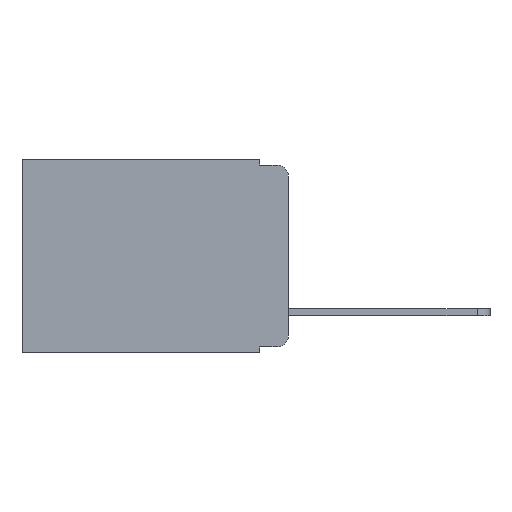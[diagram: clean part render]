
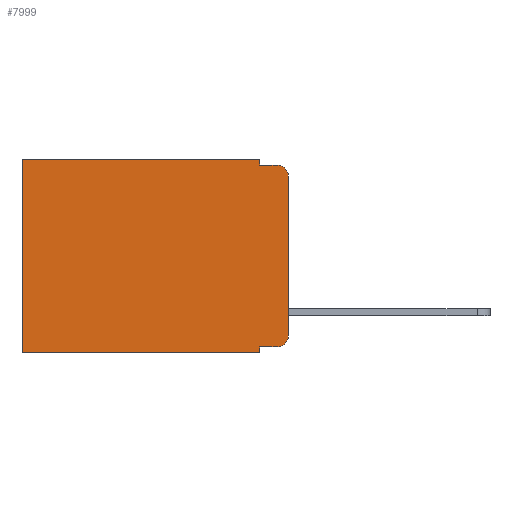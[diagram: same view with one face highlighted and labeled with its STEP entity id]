
A CAD part, left-side view. The second image highlights one B-rep face of the part: STEP entity #7999.
In plain terms, the highlighted planar face has unit normal (-1, 0, 0).
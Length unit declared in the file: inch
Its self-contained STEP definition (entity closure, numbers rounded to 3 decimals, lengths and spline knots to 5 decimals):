
#23 = CARTESIAN_POINT ( 'NONE',  ( 0.298, 0.051, 0. ) ) ;
#104 = EDGE_CURVE ( 'NONE', #6155, #2295, #5084, .T. ) ;
#171 = LINE ( 'NONE', #7430, #8221 ) ;
#211 = EDGE_CURVE ( 'NONE', #7079, #8938, #4301, .T. ) ;
#266 = DIRECTION ( 'NONE',  ( 0., 0., -1. ) ) ;
#279 = EDGE_CURVE ( 'NONE', #7079, #2295, #1635, .T. ) ;
#537 = AXIS2_PLACEMENT_3D ( 'NONE', #9211, #1673, #1945 ) ;
#915 = CARTESIAN_POINT ( 'NONE',  ( 0.298, 0.473, 0. ) ) ;
#1089 = AXIS2_PLACEMENT_3D ( 'NONE', #8195, #5437, #266 ) ;
#1116 = LINE ( 'NONE', #1208, #8933 ) ;
#1134 = ORIENTED_EDGE ( 'NONE', *, *, #9712, .F. ) ;
#1159 = DIRECTION ( 'NONE',  ( 0., 1., 0. ) ) ;
#1208 = CARTESIAN_POINT ( 'NONE',  ( 0.298, 0., 0. ) ) ;
#1389 = VERTEX_POINT ( 'NONE', #915 ) ;
#1422 = DIRECTION ( 'NONE',  ( 0., 0., -1. ) ) ;
#1485 = CARTESIAN_POINT ( 'NONE',  ( 0.298, 0.051, -0.01 ) ) ;
#1495 = ORIENTED_EDGE ( 'NONE', *, *, #211, .T. ) ;
#1497 = CARTESIAN_POINT ( 'NONE',  ( 0.298, 0.051, -0.333 ) ) ;
#1635 = LINE ( 'NONE', #7887, #9366 ) ;
#1673 = DIRECTION ( 'NONE',  ( 1., 0., 0. ) ) ;
#1716 = VECTOR ( 'NONE', #6301, 39.37008 ) ;
#1945 = DIRECTION ( 'NONE',  ( 0., 0., -1. ) ) ;
#1985 = CARTESIAN_POINT ( 'NONE',  ( 0.298, 0., -0.313 ) ) ;
#2082 = VERTEX_POINT ( 'NONE', #23 ) ;
#2113 = VECTOR ( 'NONE', #7690, 39.37008 ) ;
#2252 = EDGE_CURVE ( 'NONE', #9765, #6155, #6009, .T. ) ;
#2271 = EDGE_CURVE ( 'NONE', #1389, #5753, #5762, .T. ) ;
#2295 = VERTEX_POINT ( 'NONE', #1985 ) ;
#2302 = EDGE_CURVE ( 'NONE', #8059, #8938, #7414, .T. ) ;
#2346 = CARTESIAN_POINT ( 'NONE',  ( 0.298, 0.051, -0.333 ) ) ;
#2399 = FACE_OUTER_BOUND ( 'NONE', #6199, .T. ) ;
#2640 = CARTESIAN_POINT ( 'NONE',  ( 0.298, 0.473, 0. ) ) ;
#2781 = ORIENTED_EDGE ( 'NONE', *, *, #104, .T. ) ;
#2890 = ORIENTED_EDGE ( 'NONE', *, *, #5347, .T. ) ;
#3157 = ORIENTED_EDGE ( 'NONE', *, *, #279, .F. ) ;
#3312 = VECTOR ( 'NONE', #3568, 39.37008 ) ;
#3568 = DIRECTION ( 'NONE',  ( 0., 1., 0. ) ) ;
#3629 = VECTOR ( 'NONE', #1422, 39.37008 ) ;
#3908 = CARTESIAN_POINT ( 'NONE',  ( 0.298, 0.051, -0.343 ) ) ;
#3934 = VERTEX_POINT ( 'NONE', #3908 ) ;
#4175 = ORIENTED_EDGE ( 'NONE', *, *, #8440, .F. ) ;
#4301 = CIRCLE ( 'NONE', #1089, 0.02 ) ;
#4425 = CARTESIAN_POINT ( 'NONE',  ( 0.298, 0.02, -0.333 ) ) ;
#4896 = CARTESIAN_POINT ( 'NONE',  ( 0.298, 0.02, -0.313 ) ) ;
#5084 = CIRCLE ( 'NONE', #7551, 0.02 ) ;
#5105 = ORIENTED_EDGE ( 'NONE', *, *, #2302, .F. ) ;
#5309 = DIRECTION ( 'NONE',  ( 0., 0., -1. ) ) ;
#5347 = EDGE_CURVE ( 'NONE', #2082, #1389, #1116, .T. ) ;
#5437 = DIRECTION ( 'NONE',  ( -1., 0., 0. ) ) ;
#5528 = ORIENTED_EDGE ( 'NONE', *, *, #2271, .T. ) ;
#5541 = VECTOR ( 'NONE', #6223, 39.37008 ) ;
#5753 = VERTEX_POINT ( 'NONE', #9855 ) ;
#5762 = LINE ( 'NONE', #2640, #3629 ) ;
#5903 = LINE ( 'NONE', #9699, #2113 ) ;
#6009 = LINE ( 'NONE', #1497, #1716 ) ;
#6154 = CARTESIAN_POINT ( 'NONE',  ( 0.298, 0., -0.343 ) ) ;
#6155 = VERTEX_POINT ( 'NONE', #4425 ) ;
#6199 = EDGE_LOOP ( 'NONE', ( #3157, #1495, #5105, #1134, #2890, #5528, #6867, #4175, #6397, #2781 ) ) ;
#6223 = DIRECTION ( 'NONE',  ( 0., -1., 0. ) ) ;
#6263 = CARTESIAN_POINT ( 'NONE',  ( 0.298, 0.051, -0.01 ) ) ;
#6301 = DIRECTION ( 'NONE',  ( 0., -1., 0. ) ) ;
#6397 = ORIENTED_EDGE ( 'NONE', *, *, #2252, .T. ) ;
#6487 = DIRECTION ( 'NONE',  ( 0., 0., -1. ) ) ;
#6795 = EDGE_CURVE ( 'NONE', #3934, #5753, #8967, .T. ) ;
#6867 = ORIENTED_EDGE ( 'NONE', *, *, #6795, .F. ) ;
#7069 = DIRECTION ( 'NONE',  ( -1., 0., 0. ) ) ;
#7079 = VERTEX_POINT ( 'NONE', #8665 ) ;
#7414 = LINE ( 'NONE', #6263, #5541 ) ;
#7430 = CARTESIAN_POINT ( 'NONE',  ( 0.298, 0.051, 0. ) ) ;
#7551 = AXIS2_PLACEMENT_3D ( 'NONE', #4896, #7069, #6487 ) ;
#7690 = DIRECTION ( 'NONE',  ( 0., 0., -1. ) ) ;
#7887 = CARTESIAN_POINT ( 'NONE',  ( 0.298, 0., 0. ) ) ;
#7999 = ADVANCED_FACE ( 'NONE', ( #2399 ), #9225, .F. ) ;
#8059 = VERTEX_POINT ( 'NONE', #1485 ) ;
#8195 = CARTESIAN_POINT ( 'NONE',  ( 0.298, 0.02, -0.03 ) ) ;
#8221 = VECTOR ( 'NONE', #5309, 39.37008 ) ;
#8440 = EDGE_CURVE ( 'NONE', #9765, #3934, #171, .T. ) ;
#8665 = CARTESIAN_POINT ( 'NONE',  ( 0.298, 0., -0.03 ) ) ;
#8693 = CARTESIAN_POINT ( 'NONE',  ( 0.298, 0.02, -0.01 ) ) ;
#8933 = VECTOR ( 'NONE', #1159, 39.37008 ) ;
#8938 = VERTEX_POINT ( 'NONE', #8693 ) ;
#8967 = LINE ( 'NONE', #6154, #3312 ) ;
#9211 = CARTESIAN_POINT ( 'NONE',  ( 0.298, 0., 0. ) ) ;
#9225 = PLANE ( 'NONE',  #537 ) ;
#9366 = VECTOR ( 'NONE', #9741, 39.37008 ) ;
#9699 = CARTESIAN_POINT ( 'NONE',  ( 0.298, 0.051, 0. ) ) ;
#9712 = EDGE_CURVE ( 'NONE', #2082, #8059, #5903, .T. ) ;
#9741 = DIRECTION ( 'NONE',  ( 0., 0., -1. ) ) ;
#9765 = VERTEX_POINT ( 'NONE', #2346 ) ;
#9855 = CARTESIAN_POINT ( 'NONE',  ( 0.298, 0.473, -0.343 ) ) ;
